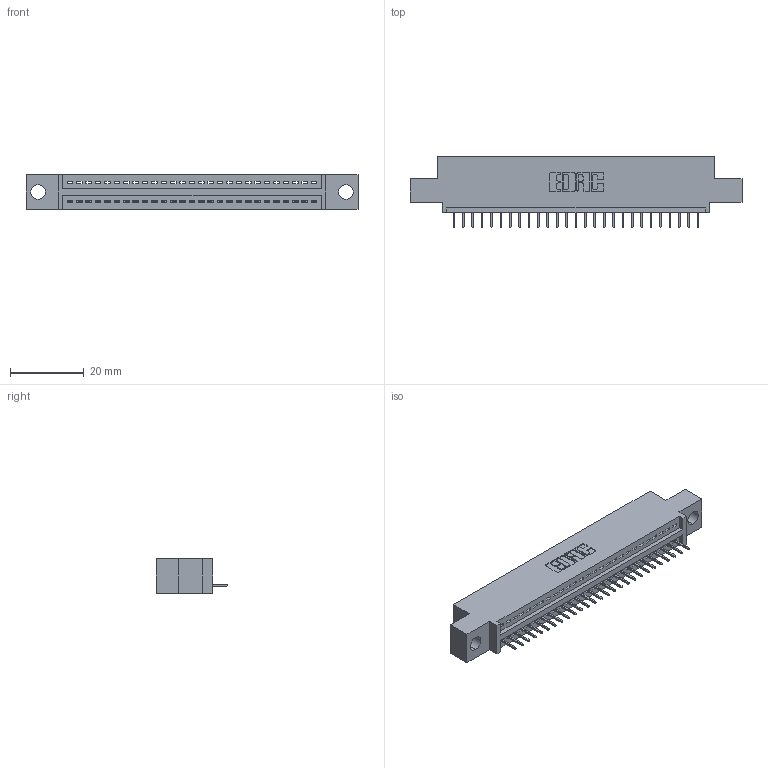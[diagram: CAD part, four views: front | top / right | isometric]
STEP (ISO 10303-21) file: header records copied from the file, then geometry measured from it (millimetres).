
FILE_DESCRIPTION (( 'STEP AP203' ), '1' );
FILE_NAME ('395-027-524-404.STEP', '2021-05-31T14:39:08', ( '' ), ( '' ), 'SwSTEP 2.0', 'SolidWorks 2020', '' );
FILE_SCHEMA (( 'CONFIG_CONTROL_DESIGN' ));
Length unit declared in the file: inch
Products named in the file (3): 345-292-001_345-293-124; 345 Part_0.110 Offset - 0.156 Dia-TI; 395-027-524-404
Assembly tree (28 placements, depth 2):
  395-027-524-404
    345 Part_0.110 Offset - 0.156 Dia-TI
    345-292-001_345-293-124  x27
Bounding box: 89.79 x 19.35 x 9.4 mm (x, y, z)
Volume: 8119.4 mm3; surface area: 10169.4 mm2
Topology: 28 solids, 28 shells, 1818 faces, 5249 edges, 3390 vertices
Faces by surface type: plane 1340, cylinder 478
Entity records: 22965 total; most frequent: CARTESIAN_POINT 3987, ORIENTED_EDGE 3946, DIRECTION 3503, EDGE_CURVE 1973, LINE 1737, VECTOR 1737, VERTEX_POINT 1310, AXIS2_PLACEMENT_3D 883
